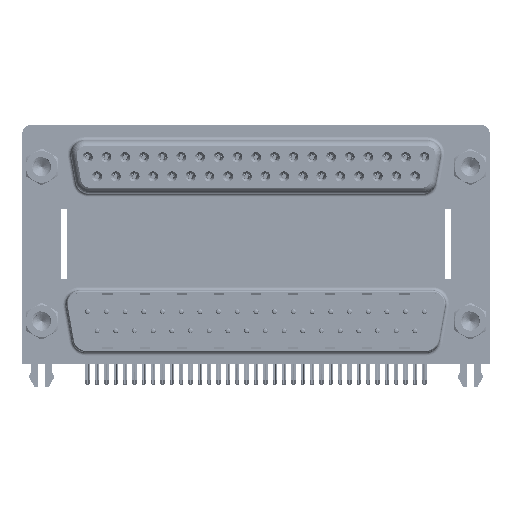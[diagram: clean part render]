
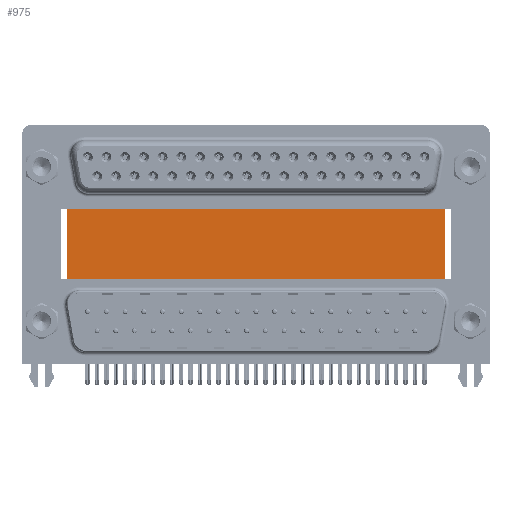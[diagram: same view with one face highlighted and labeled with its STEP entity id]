
A CAD part, top view. The second image highlights one B-rep face of the part: STEP entity #975.
In plain terms, the highlighted planar face has unit normal (0, 0, 1).
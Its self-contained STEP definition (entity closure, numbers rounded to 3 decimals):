
#975 = ADVANCED_FACE ( 'NONE', ( #31947 ), #4067, .F. ) ;
#4067 = PLANE ( 'NONE',  #27992 ) ;
#9370 = ORIENTED_EDGE ( 'NONE', *, *, #27521, .F. ) ;
#9704 = ORIENTED_EDGE ( 'NONE', *, *, #20627, .F. ) ;
#11697 = CARTESIAN_POINT ( 'NONE',  ( 59.71, -3.735, -12. ) ) ;
#12495 = CARTESIAN_POINT ( 'NONE',  ( 59.71, 16.585, -12. ) ) ;
#14241 = LINE ( 'NONE', #42077, #65354 ) ;
#16107 = DIRECTION ( 'NONE',  ( 0., 0., -1. ) ) ;
#19270 = VERTEX_POINT ( 'NONE', #47913 ) ;
#20627 = EDGE_CURVE ( 'NONE', #60399, #19270, #58558, .T. ) ;
#21425 = CARTESIAN_POINT ( 'NONE',  ( 3.79, -3.735, -12. ) ) ;
#23190 = CARTESIAN_POINT ( 'NONE',  ( 3.79, 16.585, -12. ) ) ;
#24574 = VERTEX_POINT ( 'NONE', #58050 ) ;
#27521 = EDGE_CURVE ( 'NONE', #19270, #54548, #42581, .T. ) ;
#27992 = AXIS2_PLACEMENT_3D ( 'NONE', #43956, #16107, #39064 ) ;
#29794 = VECTOR ( 'NONE', #54278, 1000. ) ;
#31947 = FACE_OUTER_BOUND ( 'NONE', #71139, .T. ) ;
#37207 = DIRECTION ( 'NONE',  ( 0., -1., 0. ) ) ;
#39064 = DIRECTION ( 'NONE',  ( -1., 0., 0. ) ) ;
#40295 = EDGE_CURVE ( 'NONE', #60399, #24574, #14241, .T. ) ;
#41299 = VECTOR ( 'NONE', #59660, 1000. ) ;
#42077 = CARTESIAN_POINT ( 'NONE',  ( 3.79, 16.585, -12. ) ) ;
#42581 = LINE ( 'NONE', #12495, #29794 ) ;
#43956 = CARTESIAN_POINT ( 'NONE',  ( 3.79, 16.585, -12. ) ) ;
#47913 = CARTESIAN_POINT ( 'NONE',  ( 59.71, 16.585, -12. ) ) ;
#47959 = CARTESIAN_POINT ( 'NONE',  ( 3.79, 16.585, -12. ) ) ;
#54278 = DIRECTION ( 'NONE',  ( 0., -1., 0. ) ) ;
#54548 = VERTEX_POINT ( 'NONE', #11697 ) ;
#55587 = ORIENTED_EDGE ( 'NONE', *, *, #59694, .T. ) ;
#58050 = CARTESIAN_POINT ( 'NONE',  ( 3.79, -3.735, -12. ) ) ;
#58558 = LINE ( 'NONE', #47959, #41299 ) ;
#59660 = DIRECTION ( 'NONE',  ( 1., 0., 0. ) ) ;
#59694 = EDGE_CURVE ( 'NONE', #24574, #54548, #61734, .T. ) ;
#60399 = VERTEX_POINT ( 'NONE', #23190 ) ;
#60997 = DIRECTION ( 'NONE',  ( 1., 0., 0. ) ) ;
#61734 = LINE ( 'NONE', #21425, #68699 ) ;
#65354 = VECTOR ( 'NONE', #37207, 1000. ) ;
#68699 = VECTOR ( 'NONE', #60997, 1000. ) ;
#68923 = ORIENTED_EDGE ( 'NONE', *, *, #40295, .T. ) ;
#71139 = EDGE_LOOP ( 'NONE', ( #55587, #9370, #9704, #68923 ) ) ;
